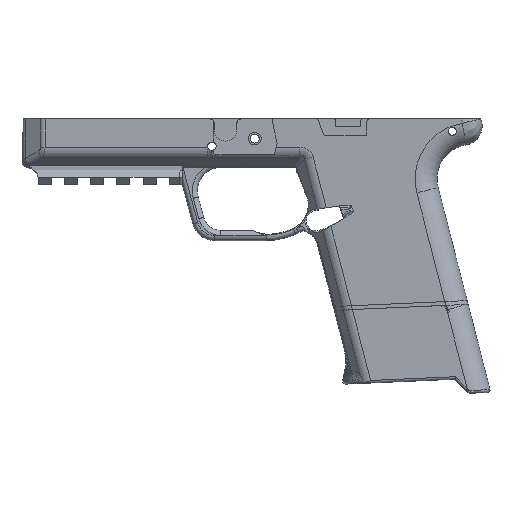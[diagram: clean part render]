
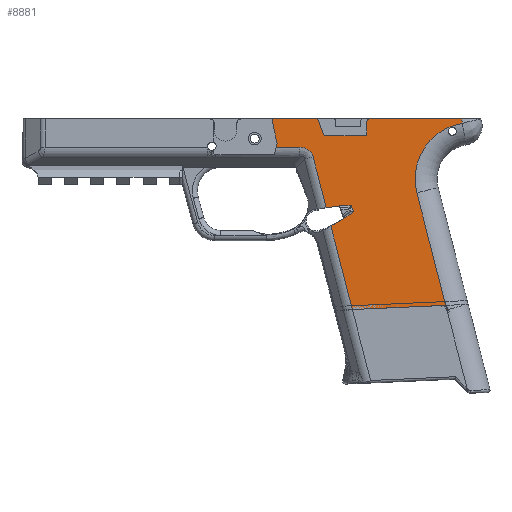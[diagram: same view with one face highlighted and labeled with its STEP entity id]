
A CAD part, left-side view. The second image highlights one B-rep face of the part: STEP entity #8881.
In plain terms, the highlighted face is planar.
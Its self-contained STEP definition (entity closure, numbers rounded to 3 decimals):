
#259=CIRCLE('',#9535,22.475);
#260=CIRCLE('',#9536,7.5);
#261=CIRCLE('',#9537,1.);
#262=CIRCLE('',#9538,1.);
#263=CIRCLE('',#9539,1.);
#264=CIRCLE('',#9540,1.);
#747=FACE_OUTER_BOUND('',#1257,.T.);
#1257=EDGE_LOOP('',(#6631,#6632,#6633,#6634,#6635,#6636,#6637,#6638,#6639,
#6640,#6641,#6642,#6643,#6644,#6645,#6646,#6647,#6648,#6649,#6650,#6651,
#6652,#6653,#6654,#6655,#6656));
#1883=LINE('',#14674,#2663);
#1885=LINE('',#14686,#2665);
#1887=LINE('',#14690,#2667);
#1898=LINE('',#14719,#2678);
#1899=LINE('',#14721,#2679);
#1900=LINE('',#14722,#2680);
#1901=LINE('',#14724,#2681);
#1902=LINE('',#14726,#2682);
#1903=LINE('',#14728,#2683);
#1904=LINE('',#14730,#2684);
#1905=LINE('',#14736,#2685);
#1906=LINE('',#14740,#2686);
#1907=LINE('',#14744,#2687);
#1908=LINE('',#14748,#2688);
#1909=LINE('',#14752,#2689);
#1910=LINE('',#14754,#2690);
#1911=LINE('',#14756,#2691);
#1912=LINE('',#14758,#2692);
#1913=LINE('',#14761,#2693);
#2663=VECTOR('',#10893,10.);
#2665=VECTOR('',#10903,10.);
#2667=VECTOR('',#10907,10.);
#2678=VECTOR('',#10928,10.);
#2679=VECTOR('',#10929,10.);
#2680=VECTOR('',#10930,10.);
#2681=VECTOR('',#10931,10.);
#2682=VECTOR('',#10932,10.);
#2683=VECTOR('',#10933,10.);
#2684=VECTOR('',#10934,10.);
#2685=VECTOR('',#10939,10.);
#2686=VECTOR('',#10942,10.);
#2687=VECTOR('',#10945,10.);
#2688=VECTOR('',#10948,10.);
#2689=VECTOR('',#10951,10.);
#2690=VECTOR('',#10952,10.);
#2691=VECTOR('',#10953,10.);
#2692=VECTOR('',#10954,10.);
#2693=VECTOR('',#10957,10.);
#3237=ELLIPSE('',#9541,10.693,7.);
#3843=VERTEX_POINT('',#14671);
#3844=VERTEX_POINT('',#14673);
#3849=VERTEX_POINT('',#14683);
#3850=VERTEX_POINT('',#14685);
#3851=VERTEX_POINT('',#14689);
#3864=VERTEX_POINT('',#14718);
#3865=VERTEX_POINT('',#14720);
#3866=VERTEX_POINT('',#14723);
#3867=VERTEX_POINT('',#14725);
#3868=VERTEX_POINT('',#14727);
#3869=VERTEX_POINT('',#14729);
#3870=VERTEX_POINT('',#14731);
#3871=VERTEX_POINT('',#14733);
#3872=VERTEX_POINT('',#14735);
#3873=VERTEX_POINT('',#14737);
#3874=VERTEX_POINT('',#14739);
#3875=VERTEX_POINT('',#14741);
#3876=VERTEX_POINT('',#14743);
#3877=VERTEX_POINT('',#14745);
#3878=VERTEX_POINT('',#14747);
#3879=VERTEX_POINT('',#14749);
#3880=VERTEX_POINT('',#14751);
#3881=VERTEX_POINT('',#14753);
#3882=VERTEX_POINT('',#14755);
#3883=VERTEX_POINT('',#14757);
#3884=VERTEX_POINT('',#14759);
#4863=EDGE_CURVE('',#3844,#3843,#1883,.T.);
#4869=EDGE_CURVE('',#3850,#3849,#1885,.T.);
#4871=EDGE_CURVE('',#3851,#3850,#1887,.T.);
#4886=EDGE_CURVE('',#3864,#3849,#1898,.T.);
#4887=EDGE_CURVE('',#3865,#3864,#1899,.T.);
#4888=EDGE_CURVE('',#3844,#3865,#1900,.T.);
#4889=EDGE_CURVE('',#3843,#3866,#1901,.T.);
#4890=EDGE_CURVE('',#3867,#3866,#1902,.T.);
#4891=EDGE_CURVE('',#3868,#3867,#1903,.T.);
#4892=EDGE_CURVE('',#3869,#3868,#1904,.T.);
#4893=EDGE_CURVE('',#3870,#3869,#259,.T.);
#4894=EDGE_CURVE('',#3871,#3870,#260,.T.);
#4895=EDGE_CURVE('',#3871,#3872,#1905,.T.);
#4896=EDGE_CURVE('',#3873,#3872,#261,.T.);
#4897=EDGE_CURVE('',#3873,#3874,#1906,.T.);
#4898=EDGE_CURVE('',#3875,#3874,#262,.T.);
#4899=EDGE_CURVE('',#3875,#3876,#1907,.T.);
#4900=EDGE_CURVE('',#3877,#3876,#263,.T.);
#4901=EDGE_CURVE('',#3878,#3877,#1908,.T.);
#4902=EDGE_CURVE('',#3879,#3878,#264,.T.);
#4903=EDGE_CURVE('',#3880,#3879,#1909,.T.);
#4904=EDGE_CURVE('',#3880,#3881,#1910,.T.);
#4905=EDGE_CURVE('',#3881,#3882,#1911,.T.);
#4906=EDGE_CURVE('',#3883,#3882,#1912,.T.);
#4907=EDGE_CURVE('',#3884,#3883,#3237,.T.);
#4908=EDGE_CURVE('',#3851,#3884,#1913,.T.);
#6631=ORIENTED_EDGE('',*,*,#4869,.T.);
#6632=ORIENTED_EDGE('',*,*,#4886,.F.);
#6633=ORIENTED_EDGE('',*,*,#4887,.F.);
#6634=ORIENTED_EDGE('',*,*,#4888,.F.);
#6635=ORIENTED_EDGE('',*,*,#4863,.T.);
#6636=ORIENTED_EDGE('',*,*,#4889,.T.);
#6637=ORIENTED_EDGE('',*,*,#4890,.F.);
#6638=ORIENTED_EDGE('',*,*,#4891,.F.);
#6639=ORIENTED_EDGE('',*,*,#4892,.F.);
#6640=ORIENTED_EDGE('',*,*,#4893,.F.);
#6641=ORIENTED_EDGE('',*,*,#4894,.F.);
#6642=ORIENTED_EDGE('',*,*,#4895,.T.);
#6643=ORIENTED_EDGE('',*,*,#4896,.F.);
#6644=ORIENTED_EDGE('',*,*,#4897,.T.);
#6645=ORIENTED_EDGE('',*,*,#4898,.F.);
#6646=ORIENTED_EDGE('',*,*,#4899,.T.);
#6647=ORIENTED_EDGE('',*,*,#4900,.F.);
#6648=ORIENTED_EDGE('',*,*,#4901,.F.);
#6649=ORIENTED_EDGE('',*,*,#4902,.F.);
#6650=ORIENTED_EDGE('',*,*,#4903,.F.);
#6651=ORIENTED_EDGE('',*,*,#4904,.T.);
#6652=ORIENTED_EDGE('',*,*,#4905,.T.);
#6653=ORIENTED_EDGE('',*,*,#4906,.F.);
#6654=ORIENTED_EDGE('',*,*,#4907,.F.);
#6655=ORIENTED_EDGE('',*,*,#4908,.F.);
#6656=ORIENTED_EDGE('',*,*,#4871,.T.);
#8565=PLANE('',#9534);
#8881=ADVANCED_FACE('',(#747),#8565,.F.);
#9534=AXIS2_PLACEMENT_3D('',#14717,#10926,#10927);
#9535=AXIS2_PLACEMENT_3D('',#14732,#10935,#10936);
#9536=AXIS2_PLACEMENT_3D('',#14734,#10937,#10938);
#9537=AXIS2_PLACEMENT_3D('',#14738,#10940,#10941);
#9538=AXIS2_PLACEMENT_3D('',#14742,#10943,#10944);
#9539=AXIS2_PLACEMENT_3D('',#14746,#10946,#10947);
#9540=AXIS2_PLACEMENT_3D('',#14750,#10949,#10950);
#9541=AXIS2_PLACEMENT_3D('',#14760,#10955,#10956);
#10893=DIRECTION('',(0.,-0.323,0.947));
#10903=DIRECTION('',(0.,-0.323,0.947));
#10907=DIRECTION('',(0.,-0.991,-0.136));
#10926=DIRECTION('center_axis',(-1.,0.,0.));
#10927=DIRECTION('ref_axis',(0.,1.,0.));
#10928=DIRECTION('',(0.,0.998,0.056));
#10929=DIRECTION('',(0.,0.323,-0.947));
#10930=DIRECTION('',(0.,-0.828,-0.56));
#10931=DIRECTION('',(0.,0.87,0.492));
#10932=DIRECTION('',(0.,0.249,-0.969));
#10933=DIRECTION('',(0.,0.999,0.044));
#10934=DIRECTION('',(0.,-0.249,0.969));
#10935=DIRECTION('center_axis',(1.,0.,0.));
#10936=DIRECTION('ref_axis',(0.,0.,1.));
#10937=DIRECTION('center_axis',(1.,0.,0.));
#10938=DIRECTION('ref_axis',(0.,-0.97,-0.244));
#10939=DIRECTION('',(0.,1.,0.));
#10940=DIRECTION('center_axis',(-1.,0.,0.));
#10941=DIRECTION('ref_axis',(0.,0.707,-0.707));
#10942=DIRECTION('',(0.,0.,1.));
#10943=DIRECTION('center_axis',(1.,0.,0.));
#10944=DIRECTION('ref_axis',(0.,-0.707,0.707));
#10945=DIRECTION('',(0.,1.,0.));
#10946=DIRECTION('center_axis',(1.,0.,0.));
#10947=DIRECTION('ref_axis',(0.,0.576,0.817));
#10948=DIRECTION('',(0.,-0.336,0.942));
#10949=DIRECTION('center_axis',(-1.,0.,0.));
#10950=DIRECTION('ref_axis',(0.,-0.576,-0.817));
#10951=DIRECTION('',(0.,-1.,0.));
#10952=DIRECTION('',(0.,-0.21,0.978));
#10953=DIRECTION('',(0.,0.21,0.978));
#10954=DIRECTION('',(0.,1.,0.));
#10955=DIRECTION('center_axis',(1.,0.,0.));
#10956=DIRECTION('ref_axis',(0.,-0.714,-0.7));
#10957=DIRECTION('',(0.,0.249,-0.969));
#14671=CARTESIAN_POINT('',(22.175,-34.01,32.318));
#14673=CARTESIAN_POINT('',(22.175,-33.995,32.275));
#14674=CARTESIAN_POINT('',(22.175,-27.197,12.322));
#14683=CARTESIAN_POINT('',(22.175,-32.296,27.288));
#14685=CARTESIAN_POINT('',(22.175,-32.284,27.253));
#14686=CARTESIAN_POINT('',(22.175,-27.197,12.322));
#14689=CARTESIAN_POINT('',(22.175,-27.009,27.98));
#14690=CARTESIAN_POINT('',(22.175,-17.622,29.272));
#14717=CARTESIAN_POINT('Origin',(22.175,-7.921,2.186));
#14718=CARTESIAN_POINT('',(22.175,-36.962,27.028));
#14719=CARTESIAN_POINT('',(22.175,-22.893,27.813));
#14720=CARTESIAN_POINT('',(22.175,-37.859,29.661));
#14721=CARTESIAN_POINT('',(22.175,-32.016,12.512));
#14722=CARTESIAN_POINT('',(22.175,-30.049,34.945));
#14723=CARTESIAN_POINT('',(22.175,-28.871,35.225));
#14724=CARTESIAN_POINT('',(22.175,-30.348,34.389));
#14725=CARTESIAN_POINT('',(22.175,-37.447,68.587));
#14726=CARTESIAN_POINT('',(22.175,-26.659,26.619));
#14727=CARTESIAN_POINT('',(22.175,-74.722,66.935));
#14728=CARTESIAN_POINT('',(22.175,-40.785,68.439));
#14729=CARTESIAN_POINT('',(22.175,-63.184,22.049));
#14730=CARTESIAN_POINT('',(22.175,-75.103,68.418));
#14731=CARTESIAN_POINT('',(22.175,-81.332,-5.728));
#14732=CARTESIAN_POINT('Origin',(22.175,-84.951,16.453));
#14733=CARTESIAN_POINT('',(22.175,-81.106,-7.556));
#14734=CARTESIAN_POINT('Origin',(22.175,-88.606,-7.556));
#14735=CARTESIAN_POINT('',(22.175,-44.284,-7.556));
#14736=CARTESIAN_POINT('',(22.175,-84.951,-7.556));
#14737=CARTESIAN_POINT('',(22.175,-43.284,-6.556));
#14738=CARTESIAN_POINT('Origin',(22.175,-44.284,-6.556));
#14739=CARTESIAN_POINT('',(22.175,-43.284,-1.806));
#14740=CARTESIAN_POINT('',(22.175,-43.284,-2.685));
#14741=CARTESIAN_POINT('',(22.175,-42.284,-0.806));
#14742=CARTESIAN_POINT('Origin',(22.175,-42.284,-1.806));
#14743=CARTESIAN_POINT('',(22.175,-26.754,-0.806));
#14744=CARTESIAN_POINT('',(22.175,-30.774,-0.806));
#14745=CARTESIAN_POINT('',(22.175,-25.812,-1.47));
#14746=CARTESIAN_POINT('Origin',(22.175,-26.754,-1.806));
#14747=CARTESIAN_POINT('',(22.175,-23.877,-6.892));
#14748=CARTESIAN_POINT('',(22.175,-23.64,-7.556));
#14749=CARTESIAN_POINT('',(22.175,-22.935,-7.556));
#14750=CARTESIAN_POINT('Origin',(22.175,-22.935,-6.556));
#14751=CARTESIAN_POINT('',(22.175,-5.3,-7.556));
#14752=CARTESIAN_POINT('',(22.175,-8.213,-7.556));
#14753=CARTESIAN_POINT('',(22.175,-7.389,2.186));
#14754=CARTESIAN_POINT('',(22.175,-6.356,-2.63));
#14755=CARTESIAN_POINT('',(22.175,-7.025,3.884));
#14756=CARTESIAN_POINT('',(22.175,-7.4,2.132));
#14757=CARTESIAN_POINT('',(22.175,-16.536,3.884));
#14758=CARTESIAN_POINT('',(22.175,33.814,3.884));
#14759=CARTESIAN_POINT('',(22.175,-21.783,7.651));
#14760=CARTESIAN_POINT('Origin',(22.175,-12.907,12.884));
#14761=CARTESIAN_POINT('',(22.175,-26.659,26.619));
